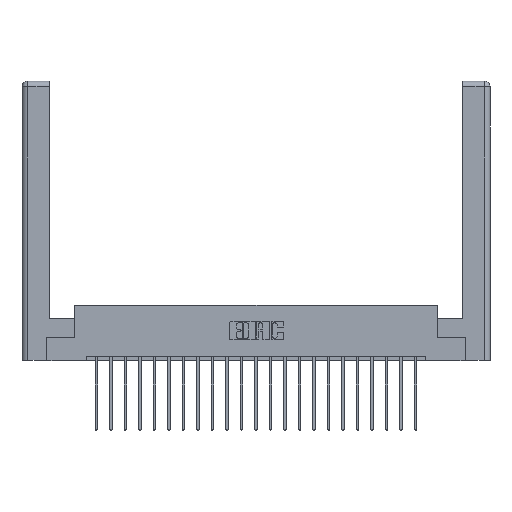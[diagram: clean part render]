
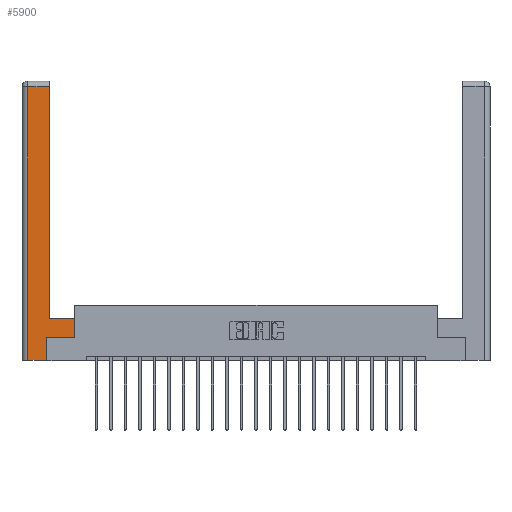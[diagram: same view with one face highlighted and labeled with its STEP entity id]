
A CAD part, top view. The second image highlights one B-rep face of the part: STEP entity #5900.
In plain terms, the highlighted planar face has unit normal (0, 0, 1).
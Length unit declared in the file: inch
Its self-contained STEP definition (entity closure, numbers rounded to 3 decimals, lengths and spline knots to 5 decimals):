
#146 = VECTOR ( 'NONE', #9860, 39.37008 ) ;
#176 = VERTEX_POINT ( 'NONE', #11252 ) ;
#314 = ORIENTED_EDGE ( 'NONE', *, *, #18662, .T. ) ;
#322 = CARTESIAN_POINT ( 'NONE',  ( 0.0615, 0., 0. ) ) ;
#423 = VECTOR ( 'NONE', #1858, 39.37008 ) ;
#712 = ORIENTED_EDGE ( 'NONE', *, *, #16856, .T. ) ;
#857 = FACE_OUTER_BOUND ( 'NONE', #5455, .T. ) ;
#1050 = CARTESIAN_POINT ( 'NONE',  ( 0.0615, 2.94, 0. ) ) ;
#1264 = AXIS2_PLACEMENT_3D ( 'NONE', #19157, #1543, #17446 ) ;
#1346 = CARTESIAN_POINT ( 'NONE',  ( 0.0615, 0., 0. ) ) ;
#1543 = DIRECTION ( 'NONE',  ( 0., 0., -1. ) ) ;
#1858 = DIRECTION ( 'NONE',  ( 0., -1., 0. ) ) ;
#2789 = ORIENTED_EDGE ( 'NONE', *, *, #21612, .T. ) ;
#3718 = CARTESIAN_POINT ( 'NONE',  ( 0.295, 2.94, 0. ) ) ;
#3885 = DIRECTION ( 'NONE',  ( -1., 0., 0. ) ) ;
#4078 = CARTESIAN_POINT ( 'NONE',  ( 0.565, 0.245, 0. ) ) ;
#4587 = LINE ( 'NONE', #20073, #7071 ) ;
#4955 = EDGE_CURVE ( 'NONE', #6125, #14732, #6653, .T. ) ;
#5455 = EDGE_LOOP ( 'NONE', ( #19741, #17801, #8349, #6825, #14943, #712, #314, #2789 ) ) ;
#5900 = ADVANCED_FACE ( 'NONE', ( #857 ), #10312, .F. ) ;
#6125 = VERTEX_POINT ( 'NONE', #9372 ) ;
#6320 = VECTOR ( 'NONE', #9441, 39.37008 ) ;
#6366 = VECTOR ( 'NONE', #7058, 39.37008 ) ;
#6653 = LINE ( 'NONE', #12588, #6366 ) ;
#6825 = ORIENTED_EDGE ( 'NONE', *, *, #11706, .T. ) ;
#7058 = DIRECTION ( 'NONE',  ( 0., 1., 0. ) ) ;
#7071 = VECTOR ( 'NONE', #9582, 39.37008 ) ;
#7850 = CARTESIAN_POINT ( 'NONE',  ( 0.565, 0.45, 0. ) ) ;
#8103 = VERTEX_POINT ( 'NONE', #1050 ) ;
#8156 = LINE ( 'NONE', #322, #423 ) ;
#8349 = ORIENTED_EDGE ( 'NONE', *, *, #18830, .T. ) ;
#9021 = VERTEX_POINT ( 'NONE', #7850 ) ;
#9372 = CARTESIAN_POINT ( 'NONE',  ( 0.265, 0., 0. ) ) ;
#9441 = DIRECTION ( 'NONE',  ( 1., 0., 0. ) ) ;
#9463 = DIRECTION ( 'NONE',  ( -1., 0., 0. ) ) ;
#9582 = DIRECTION ( 'NONE',  ( 0., 1., 0. ) ) ;
#9611 = CARTESIAN_POINT ( 'NONE',  ( 0.295, 0.45, 0. ) ) ;
#9858 = CARTESIAN_POINT ( 'NONE',  ( 0.265, 0.245, 0. ) ) ;
#9860 = DIRECTION ( 'NONE',  ( 0., 1., 0. ) ) ;
#10312 = PLANE ( 'NONE',  #1264 ) ;
#11252 = CARTESIAN_POINT ( 'NONE',  ( 0.295, 0.45, 0. ) ) ;
#11706 = EDGE_CURVE ( 'NONE', #16343, #6125, #16553, .T. ) ;
#11892 = EDGE_CURVE ( 'NONE', #176, #19328, #4587, .T. ) ;
#12521 = CARTESIAN_POINT ( 'NONE',  ( 0.265, 0., 0. ) ) ;
#12588 = CARTESIAN_POINT ( 'NONE',  ( 0.265, 0.245, 0. ) ) ;
#12808 = CARTESIAN_POINT ( 'NONE',  ( 0.0615, 2.94, 0. ) ) ;
#13055 = CARTESIAN_POINT ( 'NONE',  ( 0.565, 0.45, 0. ) ) ;
#13784 = EDGE_CURVE ( 'NONE', #19328, #8103, #18669, .T. ) ;
#14228 = CARTESIAN_POINT ( 'NONE',  ( 0.565, 0.245, 0. ) ) ;
#14732 = VERTEX_POINT ( 'NONE', #9858 ) ;
#14943 = ORIENTED_EDGE ( 'NONE', *, *, #4955, .T. ) ;
#15770 = LINE ( 'NONE', #4078, #6320 ) ;
#16343 = VERTEX_POINT ( 'NONE', #1346 ) ;
#16553 = LINE ( 'NONE', #12521, #19589 ) ;
#16594 = LINE ( 'NONE', #9611, #18804 ) ;
#16856 = EDGE_CURVE ( 'NONE', #14732, #19233, #15770, .T. ) ;
#17446 = DIRECTION ( 'NONE',  ( -1., 0., 0. ) ) ;
#17496 = DIRECTION ( 'NONE',  ( 1., 0., 0. ) ) ;
#17801 = ORIENTED_EDGE ( 'NONE', *, *, #13784, .T. ) ;
#18662 = EDGE_CURVE ( 'NONE', #19233, #9021, #22320, .T. ) ;
#18669 = LINE ( 'NONE', #12808, #21991 ) ;
#18804 = VECTOR ( 'NONE', #9463, 39.37008 ) ;
#18830 = EDGE_CURVE ( 'NONE', #8103, #16343, #8156, .T. ) ;
#19157 = CARTESIAN_POINT ( 'NONE',  ( 0., 0., 0. ) ) ;
#19233 = VERTEX_POINT ( 'NONE', #14228 ) ;
#19328 = VERTEX_POINT ( 'NONE', #3718 ) ;
#19589 = VECTOR ( 'NONE', #17496, 39.37008 ) ;
#19741 = ORIENTED_EDGE ( 'NONE', *, *, #11892, .T. ) ;
#20073 = CARTESIAN_POINT ( 'NONE',  ( 0.295, 3., 0. ) ) ;
#21612 = EDGE_CURVE ( 'NONE', #9021, #176, #16594, .T. ) ;
#21991 = VECTOR ( 'NONE', #3885, 39.37008 ) ;
#22320 = LINE ( 'NONE', #13055, #146 ) ;
